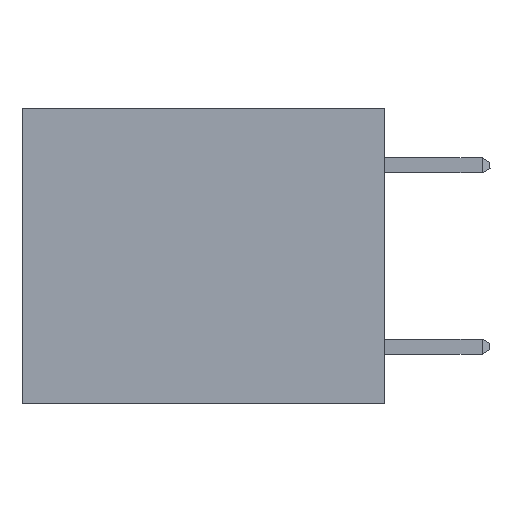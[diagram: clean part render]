
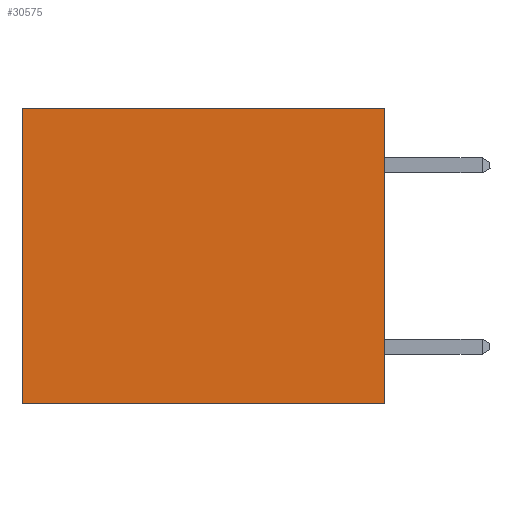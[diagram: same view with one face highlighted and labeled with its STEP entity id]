
A CAD part, left-side view. The second image highlights one B-rep face of the part: STEP entity #30575.
In plain terms, the highlighted planar face has unit normal (-1, 0, 0).
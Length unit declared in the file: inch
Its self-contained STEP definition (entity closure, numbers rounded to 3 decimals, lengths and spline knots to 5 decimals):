
#992 = CARTESIAN_POINT ( 'NONE',  ( 0.3165, 0., 0. ) ) ;
#1339 = DIRECTION ( 'NONE',  ( 1., 0., 0. ) ) ;
#1428 = FACE_OUTER_BOUND ( 'NONE', #3453, .T. ) ;
#2213 = CARTESIAN_POINT ( 'NONE',  ( 0.3165, 0.6, -0.49 ) ) ;
#2465 = VERTEX_POINT ( 'NONE', #15746 ) ;
#2916 = VERTEX_POINT ( 'NONE', #12596 ) ;
#3011 = ORIENTED_EDGE ( 'NONE', *, *, #19191, .F. ) ;
#3453 = EDGE_LOOP ( 'NONE', ( #9943, #14567, #3011, #22902 ) ) ;
#4323 = DIRECTION ( 'NONE',  ( 0., 0., -1. ) ) ;
#5280 = EDGE_CURVE ( 'NONE', #5525, #2916, #31637, .T. ) ;
#5309 = VECTOR ( 'NONE', #4323, 39.37008 ) ;
#5525 = VERTEX_POINT ( 'NONE', #17565 ) ;
#7710 = DIRECTION ( 'NONE',  ( 0., 0., -1. ) ) ;
#8552 = DIRECTION ( 'NONE',  ( 0., 1., 0. ) ) ;
#9684 = EDGE_CURVE ( 'NONE', #2916, #9796, #16050, .T. ) ;
#9796 = VERTEX_POINT ( 'NONE', #2213 ) ;
#9943 = ORIENTED_EDGE ( 'NONE', *, *, #9684, .T. ) ;
#11336 = AXIS2_PLACEMENT_3D ( 'NONE', #26727, #1339, #11806 ) ;
#11806 = DIRECTION ( 'NONE',  ( 0., 0., -1. ) ) ;
#12596 = CARTESIAN_POINT ( 'NONE',  ( 0.3165, 0.6, 0. ) ) ;
#14565 = CARTESIAN_POINT ( 'NONE',  ( 0.3165, 0.6, -0.49 ) ) ;
#14567 = ORIENTED_EDGE ( 'NONE', *, *, #24025, .F. ) ;
#14942 = LINE ( 'NONE', #27064, #29127 ) ;
#15746 = CARTESIAN_POINT ( 'NONE',  ( 0.3165, 0., -0.49 ) ) ;
#16050 = LINE ( 'NONE', #14565, #5309 ) ;
#17565 = CARTESIAN_POINT ( 'NONE',  ( 0.3165, 0., 0. ) ) ;
#19191 = EDGE_CURVE ( 'NONE', #5525, #2465, #23855, .T. ) ;
#19311 = PLANE ( 'NONE',  #11336 ) ;
#22902 = ORIENTED_EDGE ( 'NONE', *, *, #5280, .T. ) ;
#23351 = CARTESIAN_POINT ( 'NONE',  ( 0.3165, 0., -0.49 ) ) ;
#23474 = VECTOR ( 'NONE', #7710, 39.37008 ) ;
#23855 = LINE ( 'NONE', #23351, #23474 ) ;
#24025 = EDGE_CURVE ( 'NONE', #2465, #9796, #14942, .T. ) ;
#26727 = CARTESIAN_POINT ( 'NONE',  ( 0.3165, 0., -0.49 ) ) ;
#27064 = CARTESIAN_POINT ( 'NONE',  ( 0.3165, 0., -0.49 ) ) ;
#29127 = VECTOR ( 'NONE', #29675, 39.37008 ) ;
#29675 = DIRECTION ( 'NONE',  ( 0., 1., 0. ) ) ;
#30575 = ADVANCED_FACE ( 'NONE', ( #1428 ), #19311, .F. ) ;
#30841 = VECTOR ( 'NONE', #8552, 39.37008 ) ;
#31637 = LINE ( 'NONE', #992, #30841 ) ;
